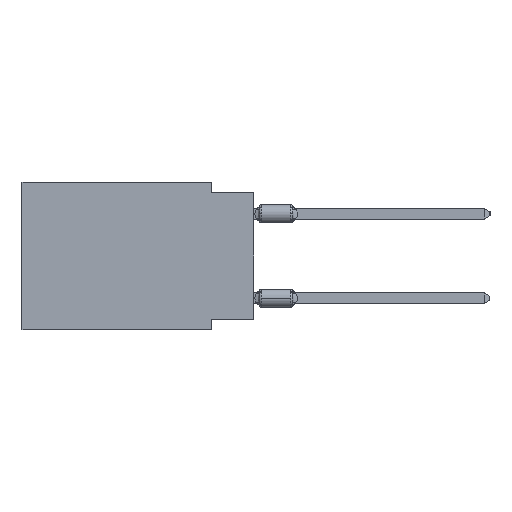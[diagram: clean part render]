
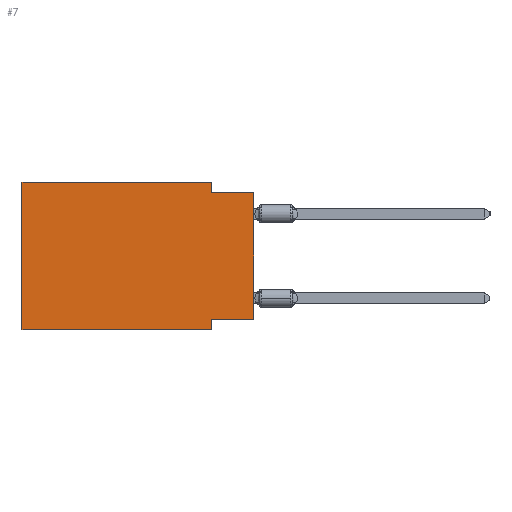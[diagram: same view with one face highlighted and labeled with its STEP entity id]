
A CAD part, left-side view. The second image highlights one B-rep face of the part: STEP entity #7.
In plain terms, the highlighted planar face has unit normal (-1, 0, 0).
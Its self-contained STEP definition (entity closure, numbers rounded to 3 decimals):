
#7 = ADVANCED_FACE ( 'NONE', ( #2299 ), #11226, .F. ) ;
#53 = CARTESIAN_POINT ( 'NONE',  ( 0., 2.54, -8.89 ) ) ;
#981 = DIRECTION ( 'NONE',  ( 0., 0., -1. ) ) ;
#2132 = LINE ( 'NONE', #19678, #27028 ) ;
#2281 = CARTESIAN_POINT ( 'NONE',  ( 0., 13.97, 0. ) ) ;
#2299 = FACE_OUTER_BOUND ( 'NONE', #20474, .T. ) ;
#2311 = DIRECTION ( 'NONE',  ( 0., -1., 0. ) ) ;
#2450 = VERTEX_POINT ( 'NONE', #10597 ) ;
#2658 = VERTEX_POINT ( 'NONE', #3537 ) ;
#3537 = CARTESIAN_POINT ( 'NONE',  ( 0., 0., -8.255 ) ) ;
#3895 = CARTESIAN_POINT ( 'NONE',  ( 0., 13.97, -8.89 ) ) ;
#5400 = VECTOR ( 'NONE', #27833, 1000. ) ;
#5748 = CARTESIAN_POINT ( 'NONE',  ( 0., 2.54, -8.89 ) ) ;
#6915 = CARTESIAN_POINT ( 'NONE',  ( 0., 13.97, 0. ) ) ;
#7201 = ORIENTED_EDGE ( 'NONE', *, *, #27872, .F. ) ;
#7988 = ORIENTED_EDGE ( 'NONE', *, *, #16709, .F. ) ;
#8565 = CARTESIAN_POINT ( 'NONE',  ( 0., 13.97, 0. ) ) ;
#9025 = LINE ( 'NONE', #29087, #11394 ) ;
#9287 = EDGE_CURVE ( 'NONE', #22159, #16541, #26798, .T. ) ;
#9329 = VECTOR ( 'NONE', #14815, 1000. ) ;
#9767 = VERTEX_POINT ( 'NONE', #15484 ) ;
#10597 = CARTESIAN_POINT ( 'NONE',  ( 0., 2.54, -8.255 ) ) ;
#10916 = DIRECTION ( 'NONE',  ( 0., 0., 1. ) ) ;
#11034 = ORIENTED_EDGE ( 'NONE', *, *, #23393, .T. ) ;
#11226 = PLANE ( 'NONE',  #22353 ) ;
#11394 = VECTOR ( 'NONE', #2311, 1000. ) ;
#11503 = LINE ( 'NONE', #22779, #25838 ) ;
#12092 = LINE ( 'NONE', #14616, #5400 ) ;
#12279 = LINE ( 'NONE', #5748, #18302 ) ;
#12639 = VERTEX_POINT ( 'NONE', #29360 ) ;
#12692 = EDGE_CURVE ( 'NONE', #9767, #24427, #11503, .T. ) ;
#12852 = EDGE_CURVE ( 'NONE', #22159, #27209, #12092, .T. ) ;
#12862 = VECTOR ( 'NONE', #26930, 1000. ) ;
#14284 = CARTESIAN_POINT ( 'NONE',  ( 0., 2.54, -0.635 ) ) ;
#14515 = CARTESIAN_POINT ( 'NONE',  ( 0., 0., -8.255 ) ) ;
#14616 = CARTESIAN_POINT ( 'NONE',  ( 0., 13.97, -8.89 ) ) ;
#14815 = DIRECTION ( 'NONE',  ( 0., 1., 0. ) ) ;
#15358 = ORIENTED_EDGE ( 'NONE', *, *, #12852, .T. ) ;
#15484 = CARTESIAN_POINT ( 'NONE',  ( 0., 2.54, 0. ) ) ;
#16541 = VERTEX_POINT ( 'NONE', #8565 ) ;
#16709 = EDGE_CURVE ( 'NONE', #24427, #12639, #19945, .T. ) ;
#17048 = LINE ( 'NONE', #14515, #9329 ) ;
#17741 = DIRECTION ( 'NONE',  ( 0., 0., 1. ) ) ;
#18302 = VECTOR ( 'NONE', #981, 1000. ) ;
#18448 = ORIENTED_EDGE ( 'NONE', *, *, #12692, .F. ) ;
#19678 = CARTESIAN_POINT ( 'NONE',  ( 0., 0., 0. ) ) ;
#19945 = LINE ( 'NONE', #22317, #12862 ) ;
#20474 = EDGE_LOOP ( 'NONE', ( #11034, #7988, #18448, #20583, #23882, #15358, #22016, #7201 ) ) ;
#20583 = ORIENTED_EDGE ( 'NONE', *, *, #23027, .F. ) ;
#20684 = VECTOR ( 'NONE', #10916, 1000. ) ;
#22016 = ORIENTED_EDGE ( 'NONE', *, *, #25347, .F. ) ;
#22159 = VERTEX_POINT ( 'NONE', #3895 ) ;
#22317 = CARTESIAN_POINT ( 'NONE',  ( 0., 0., -0.635 ) ) ;
#22353 = AXIS2_PLACEMENT_3D ( 'NONE', #6915, #29364, #24875 ) ;
#22779 = CARTESIAN_POINT ( 'NONE',  ( 0., 2.54, 0. ) ) ;
#23027 = EDGE_CURVE ( 'NONE', #16541, #9767, #9025, .T. ) ;
#23393 = EDGE_CURVE ( 'NONE', #2658, #12639, #2132, .T. ) ;
#23882 = ORIENTED_EDGE ( 'NONE', *, *, #9287, .F. ) ;
#24427 = VERTEX_POINT ( 'NONE', #14284 ) ;
#24733 = DIRECTION ( 'NONE',  ( 0., 0., -1. ) ) ;
#24875 = DIRECTION ( 'NONE',  ( 0., 0., -1. ) ) ;
#25347 = EDGE_CURVE ( 'NONE', #2450, #27209, #12279, .T. ) ;
#25838 = VECTOR ( 'NONE', #24733, 1000. ) ;
#26798 = LINE ( 'NONE', #2281, #20684 ) ;
#26930 = DIRECTION ( 'NONE',  ( 0., -1., 0. ) ) ;
#27028 = VECTOR ( 'NONE', #17741, 1000. ) ;
#27209 = VERTEX_POINT ( 'NONE', #53 ) ;
#27833 = DIRECTION ( 'NONE',  ( 0., -1., 0. ) ) ;
#27872 = EDGE_CURVE ( 'NONE', #2658, #2450, #17048, .T. ) ;
#29087 = CARTESIAN_POINT ( 'NONE',  ( 0., 13.97, 0. ) ) ;
#29360 = CARTESIAN_POINT ( 'NONE',  ( 0., 0., -0.635 ) ) ;
#29364 = DIRECTION ( 'NONE',  ( 1., 0., 0. ) ) ;
